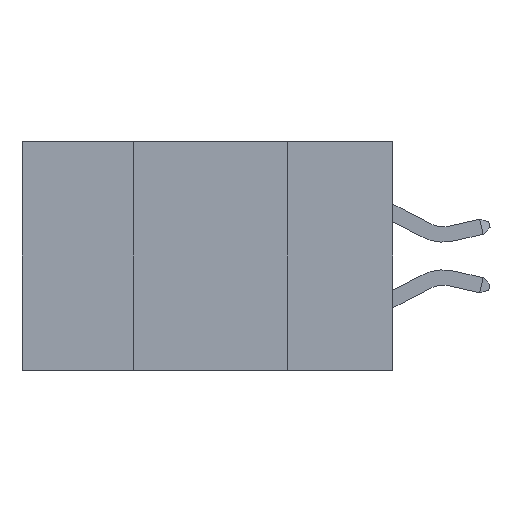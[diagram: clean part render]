
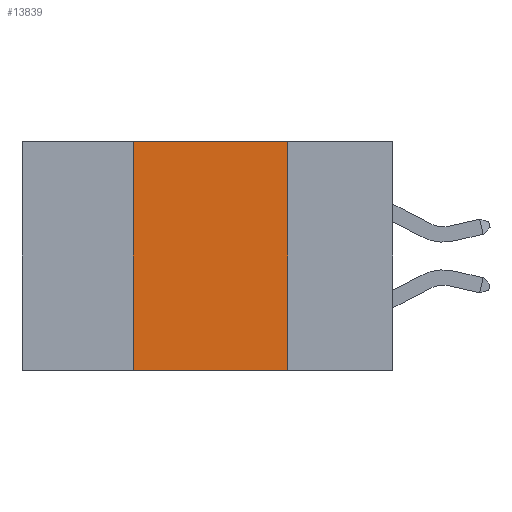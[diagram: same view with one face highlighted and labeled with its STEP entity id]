
A CAD part, left-side view. The second image highlights one B-rep face of the part: STEP entity #13839.
In plain terms, the highlighted planar face has unit normal (-1, 0, 0).
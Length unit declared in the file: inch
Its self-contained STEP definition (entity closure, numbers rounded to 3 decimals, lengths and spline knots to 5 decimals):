
#1333 = VERTEX_POINT ( 'NONE', #6276 ) ;
#1430 = EDGE_CURVE ( 'NONE', #4416, #1333, #15091, .T. ) ;
#1587 = DIRECTION ( 'NONE',  ( 0., 0., -1. ) ) ;
#1999 = EDGE_CURVE ( 'NONE', #4416, #12899, #12428, .T. ) ;
#3558 = ORIENTED_EDGE ( 'NONE', *, *, #8961, .F. ) ;
#4416 = VERTEX_POINT ( 'NONE', #13003 ) ;
#4821 = DIRECTION ( 'NONE',  ( 0., -1., 0. ) ) ;
#6120 = AXIS2_PLACEMENT_3D ( 'NONE', #9841, #18132, #1587 ) ;
#6276 = CARTESIAN_POINT ( 'NONE',  ( 0., 0.17, -0.37 ) ) ;
#6349 = CARTESIAN_POINT ( 'NONE',  ( 0., 0.6, 0. ) ) ;
#6897 = CARTESIAN_POINT ( 'NONE',  ( 0., 0.42, 0. ) ) ;
#8446 = LINE ( 'NONE', #6349, #9166 ) ;
#8961 = EDGE_CURVE ( 'NONE', #18252, #1333, #13486, .T. ) ;
#9166 = VECTOR ( 'NONE', #24384, 39.37008 ) ;
#9545 = ORIENTED_EDGE ( 'NONE', *, *, #1430, .T. ) ;
#9841 = CARTESIAN_POINT ( 'NONE',  ( 0., 0.6, 0. ) ) ;
#11526 = DIRECTION ( 'NONE',  ( 0., 0., -1. ) ) ;
#12428 = LINE ( 'NONE', #6897, #17772 ) ;
#12899 = VERTEX_POINT ( 'NONE', #21019 ) ;
#13003 = CARTESIAN_POINT ( 'NONE',  ( 0., 0.42, -0.37 ) ) ;
#13486 = LINE ( 'NONE', #15608, #15633 ) ;
#13839 = ADVANCED_FACE ( 'NONE', ( #23651 ), #19599, .F. ) ;
#14931 = DIRECTION ( 'NONE',  ( 0., 0., 1. ) ) ;
#15091 = LINE ( 'NONE', #19181, #15680 ) ;
#15450 = EDGE_LOOP ( 'NONE', ( #3558, #21258, #16846, #9545 ) ) ;
#15608 = CARTESIAN_POINT ( 'NONE',  ( 0., 0.17, 0. ) ) ;
#15633 = VECTOR ( 'NONE', #11526, 39.37008 ) ;
#15680 = VECTOR ( 'NONE', #4821, 39.37008 ) ;
#15757 = CARTESIAN_POINT ( 'NONE',  ( 0., 0.17, 0. ) ) ;
#16846 = ORIENTED_EDGE ( 'NONE', *, *, #1999, .F. ) ;
#17772 = VECTOR ( 'NONE', #14931, 39.37008 ) ;
#18132 = DIRECTION ( 'NONE',  ( 1., 0., 0. ) ) ;
#18252 = VERTEX_POINT ( 'NONE', #15757 ) ;
#19181 = CARTESIAN_POINT ( 'NONE',  ( 0., 0.6, -0.37 ) ) ;
#19599 = PLANE ( 'NONE',  #6120 ) ;
#21019 = CARTESIAN_POINT ( 'NONE',  ( 0., 0.42, 0. ) ) ;
#21258 = ORIENTED_EDGE ( 'NONE', *, *, #21854, .F. ) ;
#21854 = EDGE_CURVE ( 'NONE', #12899, #18252, #8446, .T. ) ;
#23651 = FACE_OUTER_BOUND ( 'NONE', #15450, .T. ) ;
#24384 = DIRECTION ( 'NONE',  ( 0., -1., 0. ) ) ;
